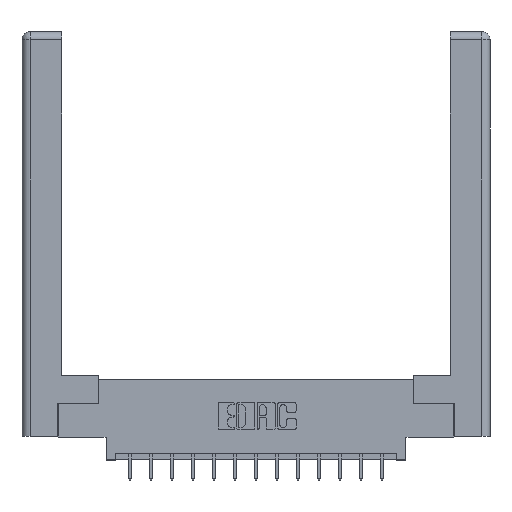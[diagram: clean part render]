
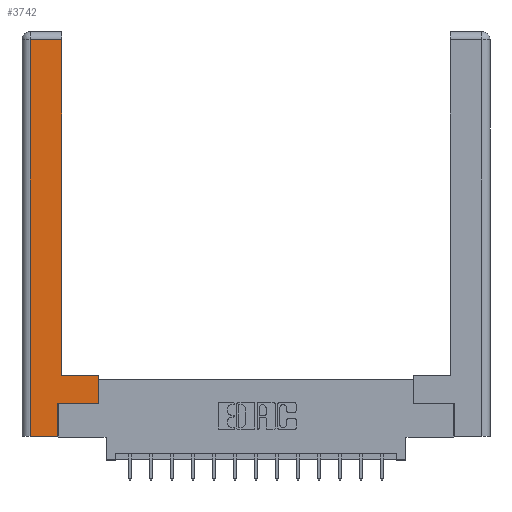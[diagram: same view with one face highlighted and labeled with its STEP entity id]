
A CAD part, top view. The second image highlights one B-rep face of the part: STEP entity #3742.
In plain terms, the highlighted planar face has unit normal (0, 0, 1).
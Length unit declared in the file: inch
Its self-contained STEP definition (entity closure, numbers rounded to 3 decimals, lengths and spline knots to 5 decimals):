
#103 = VERTEX_POINT ( 'NONE', #863 ) ;
#150 = CARTESIAN_POINT ( 'NONE',  ( 0.265, 0., 0. ) ) ;
#224 = LINE ( 'NONE', #14248, #7474 ) ;
#484 = DIRECTION ( 'NONE',  ( 1., 0., 0. ) ) ;
#570 = DIRECTION ( 'NONE',  ( 0., 1., 0. ) ) ;
#578 = LINE ( 'NONE', #1353, #10459 ) ;
#863 = CARTESIAN_POINT ( 'NONE',  ( 0.265, 0.245, 0. ) ) ;
#1314 = EDGE_CURVE ( 'NONE', #7472, #9828, #578, .T. ) ;
#1353 = CARTESIAN_POINT ( 'NONE',  ( 0.0615, 2.94, 0. ) ) ;
#1643 = LINE ( 'NONE', #4401, #11313 ) ;
#1683 = VECTOR ( 'NONE', #6391, 39.37008 ) ;
#2177 = ORIENTED_EDGE ( 'NONE', *, *, #8148, .T. ) ;
#2308 = VECTOR ( 'NONE', #570, 39.37008 ) ;
#2326 = LINE ( 'NONE', #3192, #14973 ) ;
#2402 = CARTESIAN_POINT ( 'NONE',  ( 0.295, 3., 0. ) ) ;
#2481 = CARTESIAN_POINT ( 'NONE',  ( 0.565, 0.245, 0. ) ) ;
#3084 = PLANE ( 'NONE',  #12563 ) ;
#3192 = CARTESIAN_POINT ( 'NONE',  ( 0.295, 0.45, 0. ) ) ;
#3485 = ORIENTED_EDGE ( 'NONE', *, *, #14820, .T. ) ;
#3742 = ADVANCED_FACE ( 'NONE', ( #11278 ), #3084, .F. ) ;
#3889 = LINE ( 'NONE', #2402, #1683 ) ;
#4242 = CARTESIAN_POINT ( 'NONE',  ( 0., 0., 0. ) ) ;
#4401 = CARTESIAN_POINT ( 'NONE',  ( 0.565, 0.245, 0. ) ) ;
#4699 = ORIENTED_EDGE ( 'NONE', *, *, #10264, .T. ) ;
#6043 = CARTESIAN_POINT ( 'NONE',  ( 0.0615, 2.94, 0. ) ) ;
#6391 = DIRECTION ( 'NONE',  ( 0., 1., 0. ) ) ;
#6719 = CARTESIAN_POINT ( 'NONE',  ( 0.295, 2.94, 0. ) ) ;
#7032 = CARTESIAN_POINT ( 'NONE',  ( 0.265, 0.245, 0. ) ) ;
#7316 = ORIENTED_EDGE ( 'NONE', *, *, #8342, .T. ) ;
#7472 = VERTEX_POINT ( 'NONE', #6719 ) ;
#7474 = VECTOR ( 'NONE', #9049, 39.37008 ) ;
#7762 = VERTEX_POINT ( 'NONE', #13659 ) ;
#8139 = VERTEX_POINT ( 'NONE', #2481 ) ;
#8148 = EDGE_CURVE ( 'NONE', #7762, #7472, #3889, .T. ) ;
#8323 = LINE ( 'NONE', #11969, #10343 ) ;
#8342 = EDGE_CURVE ( 'NONE', #8139, #10558, #8323, .T. ) ;
#8412 = ORIENTED_EDGE ( 'NONE', *, *, #14301, .T. ) ;
#8793 = CARTESIAN_POINT ( 'NONE',  ( 0.0615, 0., 0. ) ) ;
#9049 = DIRECTION ( 'NONE',  ( 0., -1., 0. ) ) ;
#9151 = EDGE_CURVE ( 'NONE', #103, #8139, #1643, .T. ) ;
#9575 = LINE ( 'NONE', #7032, #2308 ) ;
#9828 = VERTEX_POINT ( 'NONE', #6043 ) ;
#10264 = EDGE_CURVE ( 'NONE', #9828, #12532, #224, .T. ) ;
#10271 = EDGE_CURVE ( 'NONE', #12532, #16385, #11707, .T. ) ;
#10343 = VECTOR ( 'NONE', #15878, 39.37008 ) ;
#10371 = DIRECTION ( 'NONE',  ( -1., 0., 0. ) ) ;
#10459 = VECTOR ( 'NONE', #10371, 39.37008 ) ;
#10517 = CARTESIAN_POINT ( 'NONE',  ( 0.565, 0.45, 0. ) ) ;
#10558 = VERTEX_POINT ( 'NONE', #10517 ) ;
#11278 = FACE_OUTER_BOUND ( 'NONE', #15302, .T. ) ;
#11311 = VECTOR ( 'NONE', #484, 39.37008 ) ;
#11313 = VECTOR ( 'NONE', #13587, 39.37008 ) ;
#11707 = LINE ( 'NONE', #150, #11311 ) ;
#11969 = CARTESIAN_POINT ( 'NONE',  ( 0.565, 0.45, 0. ) ) ;
#12532 = VERTEX_POINT ( 'NONE', #8793 ) ;
#12563 = AXIS2_PLACEMENT_3D ( 'NONE', #4242, #13135, #13246 ) ;
#13135 = DIRECTION ( 'NONE',  ( 0., 0., -1. ) ) ;
#13229 = CARTESIAN_POINT ( 'NONE',  ( 0.265, 0., 0. ) ) ;
#13246 = DIRECTION ( 'NONE',  ( -1., 0., 0. ) ) ;
#13481 = ORIENTED_EDGE ( 'NONE', *, *, #1314, .T. ) ;
#13587 = DIRECTION ( 'NONE',  ( 1., 0., 0. ) ) ;
#13659 = CARTESIAN_POINT ( 'NONE',  ( 0.295, 0.45, 0. ) ) ;
#14025 = ORIENTED_EDGE ( 'NONE', *, *, #10271, .T. ) ;
#14248 = CARTESIAN_POINT ( 'NONE',  ( 0.0615, 0., 0. ) ) ;
#14301 = EDGE_CURVE ( 'NONE', #10558, #7762, #2326, .T. ) ;
#14820 = EDGE_CURVE ( 'NONE', #16385, #103, #9575, .T. ) ;
#14973 = VECTOR ( 'NONE', #16197, 39.37008 ) ;
#15302 = EDGE_LOOP ( 'NONE', ( #2177, #13481, #4699, #14025, #3485, #16483, #7316, #8412 ) ) ;
#15878 = DIRECTION ( 'NONE',  ( 0., 1., 0. ) ) ;
#16197 = DIRECTION ( 'NONE',  ( -1., 0., 0. ) ) ;
#16385 = VERTEX_POINT ( 'NONE', #13229 ) ;
#16483 = ORIENTED_EDGE ( 'NONE', *, *, #9151, .T. ) ;
